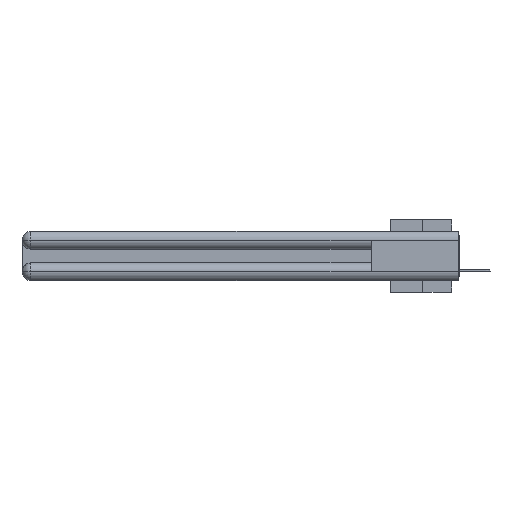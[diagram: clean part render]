
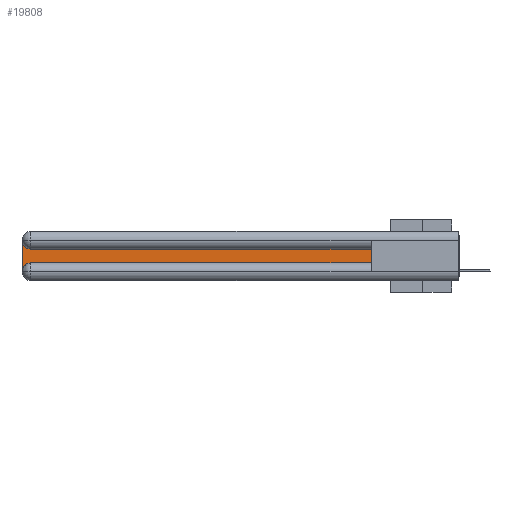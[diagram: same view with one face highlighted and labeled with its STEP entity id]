
A CAD part, left-side view. The second image highlights one B-rep face of the part: STEP entity #19808.
In plain terms, the highlighted planar face has unit normal (-1, 0, 0).
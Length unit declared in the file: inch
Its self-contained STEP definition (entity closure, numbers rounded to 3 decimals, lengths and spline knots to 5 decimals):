
#675 = ORIENTED_EDGE ( 'NONE', *, *, #5222, .T. ) ;
#699 = CARTESIAN_POINT ( 'NONE',  ( 0.075, 0.6, -0.1225 ) ) ;
#1615 = VERTEX_POINT ( 'NONE', #3974 ) ;
#1767 = DIRECTION ( 'NONE',  ( 0., 0., -1. ) ) ;
#1790 = CIRCLE ( 'NONE', #20525, 0.06 ) ;
#3974 = CARTESIAN_POINT ( 'NONE',  ( 0.075, 2.94, -0.2175 ) ) ;
#4018 = LINE ( 'NONE', #20523, #20348 ) ;
#5222 = EDGE_CURVE ( 'NONE', #1615, #20341, #10862, .T. ) ;
#5513 = VERTEX_POINT ( 'NONE', #25584 ) ;
#6539 = LINE ( 'NONE', #23691, #28456 ) ;
#6628 = EDGE_CURVE ( 'NONE', #5513, #1615, #1790, .T. ) ;
#6741 = FACE_OUTER_BOUND ( 'NONE', #23662, .T. ) ;
#7307 = ORIENTED_EDGE ( 'NONE', *, *, #6628, .T. ) ;
#8213 = CIRCLE ( 'NONE', #25957, 0.06 ) ;
#8790 = CARTESIAN_POINT ( 'NONE',  ( 0.075, 0.6, -0.2175 ) ) ;
#9052 = ORIENTED_EDGE ( 'NONE', *, *, #18911, .T. ) ;
#9214 = VERTEX_POINT ( 'NONE', #30983 ) ;
#9591 = DIRECTION ( 'NONE',  ( 0., 0., -1. ) ) ;
#10862 = LINE ( 'NONE', #8790, #29626 ) ;
#11824 = PLANE ( 'NONE',  #17636 ) ;
#13826 = CARTESIAN_POINT ( 'NONE',  ( 0.075, 2.94, -0.2775 ) ) ;
#14676 = CARTESIAN_POINT ( 'NONE',  ( 0.075, 3., -0.1225 ) ) ;
#14944 = CARTESIAN_POINT ( 'NONE',  ( 0.075, 0.6, -0.2175 ) ) ;
#15894 = ORIENTED_EDGE ( 'NONE', *, *, #18685, .T. ) ;
#16266 = CARTESIAN_POINT ( 'NONE',  ( 0.075, 2.94, -0.1225 ) ) ;
#16692 = DIRECTION ( 'NONE',  ( 0., 0., -1. ) ) ;
#16780 = VECTOR ( 'NONE', #16692, 39.37008 ) ;
#17636 = AXIS2_PLACEMENT_3D ( 'NONE', #14676, #19436, #9591 ) ;
#17976 = DIRECTION ( 'NONE',  ( 0., 0., 1. ) ) ;
#18599 = DIRECTION ( 'NONE',  ( 0., 1., 0. ) ) ;
#18685 = EDGE_CURVE ( 'NONE', #20341, #24763, #4018, .T. ) ;
#18911 = EDGE_CURVE ( 'NONE', #9214, #5513, #28452, .T. ) ;
#19436 = DIRECTION ( 'NONE',  ( 1., 0., 0. ) ) ;
#19808 = ADVANCED_FACE ( 'NONE', ( #6741 ), #11824, .F. ) ;
#20341 = VERTEX_POINT ( 'NONE', #14944 ) ;
#20348 = VECTOR ( 'NONE', #17976, 39.37008 ) ;
#20523 = CARTESIAN_POINT ( 'NONE',  ( 0.075, 0.6, -0.2175 ) ) ;
#20525 = AXIS2_PLACEMENT_3D ( 'NONE', #13826, #20829, #1767 ) ;
#20829 = DIRECTION ( 'NONE',  ( 1., 0., 0. ) ) ;
#21187 = DIRECTION ( 'NONE',  ( 0., -1., 0. ) ) ;
#21639 = ORIENTED_EDGE ( 'NONE', *, *, #27237, .T. ) ;
#23662 = EDGE_LOOP ( 'NONE', ( #21639, #29185, #9052, #7307, #675, #15894 ) ) ;
#23691 = CARTESIAN_POINT ( 'NONE',  ( 0.075, 0.6, -0.1225 ) ) ;
#24763 = VERTEX_POINT ( 'NONE', #699 ) ;
#25584 = CARTESIAN_POINT ( 'NONE',  ( 0.075, 3., -0.2775 ) ) ;
#25951 = DIRECTION ( 'NONE',  ( 0., 0., -1. ) ) ;
#25957 = AXIS2_PLACEMENT_3D ( 'NONE', #28495, #28331, #25951 ) ;
#26209 = CARTESIAN_POINT ( 'NONE',  ( 0.075, 3., -0.2175 ) ) ;
#27237 = EDGE_CURVE ( 'NONE', #24763, #29156, #6539, .T. ) ;
#28117 = EDGE_CURVE ( 'NONE', #29156, #9214, #8213, .T. ) ;
#28331 = DIRECTION ( 'NONE',  ( 1., 0., 0. ) ) ;
#28452 = LINE ( 'NONE', #26209, #16780 ) ;
#28456 = VECTOR ( 'NONE', #18599, 39.37008 ) ;
#28495 = CARTESIAN_POINT ( 'NONE',  ( 0.075, 2.94, -0.0625 ) ) ;
#29156 = VERTEX_POINT ( 'NONE', #16266 ) ;
#29185 = ORIENTED_EDGE ( 'NONE', *, *, #28117, .T. ) ;
#29626 = VECTOR ( 'NONE', #21187, 39.37008 ) ;
#30983 = CARTESIAN_POINT ( 'NONE',  ( 0.075, 3., -0.0625 ) ) ;
